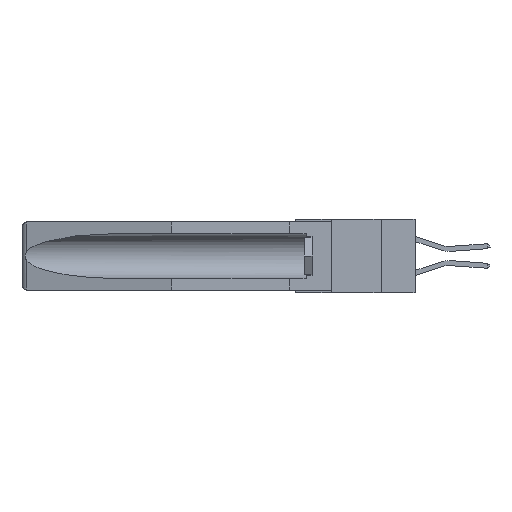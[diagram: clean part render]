
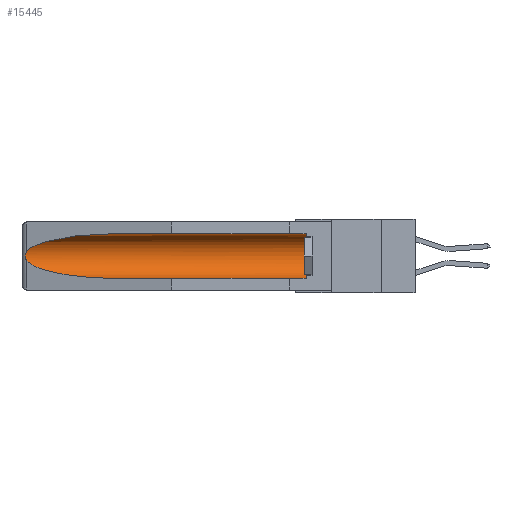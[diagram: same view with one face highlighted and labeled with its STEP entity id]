
A CAD part, left-side view. The second image highlights one B-rep face of the part: STEP entity #15445.
In plain terms, the highlighted cylindrical face has radius 2.857 mm (diameter 5.715 mm), a partial arc.
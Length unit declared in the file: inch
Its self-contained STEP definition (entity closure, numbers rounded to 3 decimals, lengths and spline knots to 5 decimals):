
#180 = DIRECTION ( 'NONE',  ( 0., 1., 0. ) ) ;
#460 = CARTESIAN_POINT ( 'NONE',  ( 0.2675, 1.53308, -0.17534 ) ) ;
#1201 = AXIS2_PLACEMENT_3D ( 'NONE', #9048, #11803, #29819 ) ;
#1693 = VECTOR ( 'NONE', #9694, 39.37008 ) ;
#1960 = CIRCLE ( 'NONE', #1201, 0.1125 ) ;
#2877 = EDGE_CURVE ( 'NONE', #20546, #28174, #11193, .T. ) ;
#3585 = CARTESIAN_POINT ( 'NONE',  ( 0.26597, 1.52961, -0.15275 ) ) ;
#3761 = EDGE_LOOP ( 'NONE', ( #24602, #13904, #9278, #20128, #15954, #20858 ) ) ;
#3921 = CARTESIAN_POINT ( 'NONE',  ( 0.2673, 1.53269, -0.17917 ) ) ;
#5635 = VERTEX_POINT ( 'NONE', #9968 ) ;
#5818 = CARTESIAN_POINT ( 'NONE',  ( 0.155, -0.30754, -0.1715 ) ) ;
#6128 = CARTESIAN_POINT ( 'NONE',  ( 0.26537, 1.52718, -0.14972 ) ) ;
#6132 = CARTESIAN_POINT ( 'NONE',  ( 0.155, 1.07973, -0.284 ) ) ;
#6622 = CARTESIAN_POINT ( 'NONE',  ( 0.155, -0.30754, -0.059 ) ) ;
#6810 = LINE ( 'NONE', #6622, #33865 ) ;
#7960 = CARTESIAN_POINT ( 'NONE',  ( 0.25451, 1.48313, -0.24835 ) ) ;
#9048 = CARTESIAN_POINT ( 'NONE',  ( 0.155, 0.126, -0.1715 ) ) ;
#9234 = DIRECTION ( 'NONE',  ( 0., 1., 0. ) ) ;
#9278 = ORIENTED_EDGE ( 'NONE', *, *, #12866, .T. ) ;
#9694 = DIRECTION ( 'NONE',  ( 0., 1., 0. ) ) ;
#9773 = VERTEX_POINT ( 'NONE', #33788 ) ;
#9968 = CARTESIAN_POINT ( 'NONE',  ( 0.155, 0.126, -0.059 ) ) ;
#11193 = B_SPLINE_CURVE_WITH_KNOTS ( 'NONE', 3,
 ( #32107, #3585, #26949, #29277, #31879, #460, #3921, #27298, #24882, #30269 ),
 .UNSPECIFIED., .F., .F.,
 ( 4, 2, 2, 2, 4 ),
 ( 0., 0.00029, 0.00058, 0.00087, 0.00117 ),
 .UNSPECIFIED. ) ;
#11206 = CARTESIAN_POINT ( 'NONE',  ( 0.21114, 1.30732, -0.059 ) ) ;
#11512 = EDGE_CURVE ( 'NONE', #5635, #20101, #6810, .T. ) ;
#11803 = DIRECTION ( 'NONE',  ( 0., -1., 0. ) ) ;
#12343 = CARTESIAN_POINT ( 'NONE',  ( 0.155, -0.30754, -0.284 ) ) ;
#12841 = CARTESIAN_POINT ( 'NONE',  ( 0.25451, 1.48313, -0.09465 ) ) ;
#12866 = EDGE_CURVE ( 'NONE', #28174, #9773, #26552, .T. ) ;
#13904 = ORIENTED_EDGE ( 'NONE', *, *, #2877, .T. ) ;
#13999 = LINE ( 'NONE', #12343, #1693 ) ;
#15445 = ADVANCED_FACE ( 'NONE', ( #18422 ), #28735, .F. ) ;
#15752 = CARTESIAN_POINT ( 'NONE',  ( 0.26537, 1.52718, -0.19328 ) ) ;
#15954 = ORIENTED_EDGE ( 'NONE', *, *, #33548, .T. ) ;
#16273 = CARTESIAN_POINT ( 'NONE',  ( 0.26537, 1.52718, -0.14972 ) ) ;
#18422 = FACE_OUTER_BOUND ( 'NONE', #3761, .T. ) ;
#18976 = EDGE_CURVE ( 'NONE', #20101, #20546, #26971, .T. ) ;
#20101 = VERTEX_POINT ( 'NONE', #32651 ) ;
#20128 = ORIENTED_EDGE ( 'NONE', *, *, #24108, .F. ) ;
#20546 = VERTEX_POINT ( 'NONE', #6128 ) ;
#20858 = ORIENTED_EDGE ( 'NONE', *, *, #11512, .T. ) ;
#21650 = AXIS2_PLACEMENT_3D ( 'NONE', #5818, #180, #24129 ) ;
#24108 = EDGE_CURVE ( 'NONE', #24999, #9773, #13999, .T. ) ;
#24129 = DIRECTION ( 'NONE',  ( 0., 0., 1. ) ) ;
#24545 = CARTESIAN_POINT ( 'NONE',  ( 0.26537, 1.52718, -0.19328 ) ) ;
#24602 = ORIENTED_EDGE ( 'NONE', *, *, #18976, .T. ) ;
#24882 = CARTESIAN_POINT ( 'NONE',  ( 0.26597, 1.5296, -0.19026 ) ) ;
#24999 = VERTEX_POINT ( 'NONE', #26496 ) ;
#26496 = CARTESIAN_POINT ( 'NONE',  ( 0.155, 0.126, -0.284 ) ) ;
#26552 =( BOUNDED_CURVE ( )  B_SPLINE_CURVE ( 3, ( #15752, #7960, #29395, #6132 ),
 .UNSPECIFIED., .F., .F. ) 
 B_SPLINE_CURVE_WITH_KNOTS ( ( 4, 4 ),
 ( 0.1948, 1.5708 ),
 .UNSPECIFIED. ) 
 CURVE ( )  GEOMETRIC_REPRESENTATION_ITEM ( )  RATIONAL_B_SPLINE_CURVE ( ( 1., 0.848, 0.848, 1. ) ) 
 REPRESENTATION_ITEM ( '' )  );
#26922 = CARTESIAN_POINT ( 'NONE',  ( 0.155, 1.07973, -0.059 ) ) ;
#26949 = CARTESIAN_POINT ( 'NONE',  ( 0.26654, 1.53092, -0.15636 ) ) ;
#26971 =( BOUNDED_CURVE ( )  B_SPLINE_CURVE ( 3, ( #26922, #11206, #12841, #16273 ),
 .UNSPECIFIED., .F., .F. ) 
 B_SPLINE_CURVE_WITH_KNOTS ( ( 4, 4 ),
 ( 4.71239, 6.08839 ),
 .UNSPECIFIED. ) 
 CURVE ( )  GEOMETRIC_REPRESENTATION_ITEM ( )  RATIONAL_B_SPLINE_CURVE ( ( 1., 0.848, 0.848, 1. ) ) 
 REPRESENTATION_ITEM ( '' )  );
#27298 = CARTESIAN_POINT ( 'NONE',  ( 0.26655, 1.53094, -0.18657 ) ) ;
#28174 = VERTEX_POINT ( 'NONE', #24545 ) ;
#28735 = CYLINDRICAL_SURFACE ( 'NONE', #21650, 0.1125 ) ;
#29277 = CARTESIAN_POINT ( 'NONE',  ( 0.2673, 1.5327, -0.16383 ) ) ;
#29395 = CARTESIAN_POINT ( 'NONE',  ( 0.21114, 1.30732, -0.284 ) ) ;
#29819 = DIRECTION ( 'NONE',  ( 0., 0., 1. ) ) ;
#30269 = CARTESIAN_POINT ( 'NONE',  ( 0.26537, 1.52718, -0.19328 ) ) ;
#31879 = CARTESIAN_POINT ( 'NONE',  ( 0.2675, 1.53308, -0.16763 ) ) ;
#32107 = CARTESIAN_POINT ( 'NONE',  ( 0.26537, 1.52718, -0.14972 ) ) ;
#32651 = CARTESIAN_POINT ( 'NONE',  ( 0.155, 1.07973, -0.059 ) ) ;
#33548 = EDGE_CURVE ( 'NONE', #24999, #5635, #1960, .T. ) ;
#33788 = CARTESIAN_POINT ( 'NONE',  ( 0.155, 1.07973, -0.284 ) ) ;
#33865 = VECTOR ( 'NONE', #9234, 39.37008 ) ;
